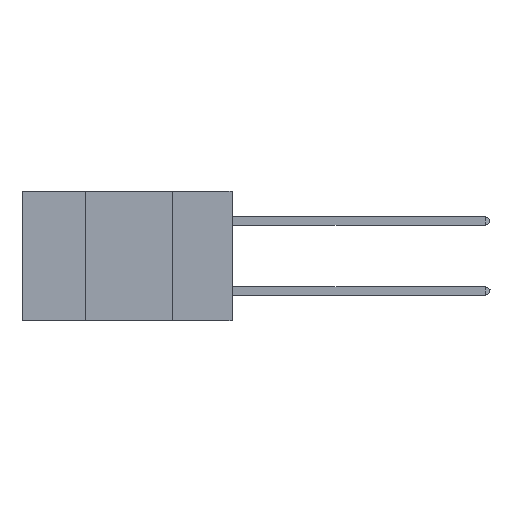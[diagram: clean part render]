
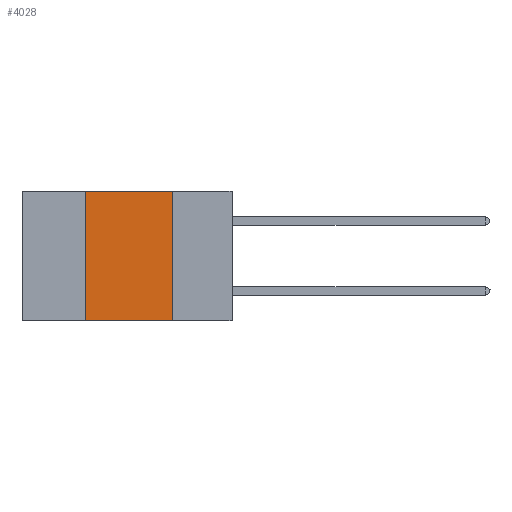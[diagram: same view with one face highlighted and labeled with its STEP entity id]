
A CAD part, left-side view. The second image highlights one B-rep face of the part: STEP entity #4028.
In plain terms, the highlighted planar face has unit normal (-1, 0, 0).
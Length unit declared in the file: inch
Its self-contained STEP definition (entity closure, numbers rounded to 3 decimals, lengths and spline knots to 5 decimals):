
#458 = DIRECTION ( 'NONE',  ( 0., -1., 0. ) ) ;
#980 = CARTESIAN_POINT ( 'NONE',  ( 0., 0.17, 0. ) ) ;
#1110 = DIRECTION ( 'NONE',  ( 0., 0., -1. ) ) ;
#1674 = AXIS2_PLACEMENT_3D ( 'NONE', #3678, #12924, #1110 ) ;
#2007 = ORIENTED_EDGE ( 'NONE', *, *, #4683, .F. ) ;
#3109 = CARTESIAN_POINT ( 'NONE',  ( 0., 0.6, -0.37 ) ) ;
#3633 = CARTESIAN_POINT ( 'NONE',  ( 0., 0.6, 0. ) ) ;
#3663 = VERTEX_POINT ( 'NONE', #13296 ) ;
#3672 = DIRECTION ( 'NONE',  ( 0., 0., -1. ) ) ;
#3678 = CARTESIAN_POINT ( 'NONE',  ( 0., 0.6, 0. ) ) ;
#3947 = DIRECTION ( 'NONE',  ( 0., 0., 1. ) ) ;
#4014 = DIRECTION ( 'NONE',  ( 0., -1., 0. ) ) ;
#4028 = ADVANCED_FACE ( 'NONE', ( #15529 ), #5142, .F. ) ;
#4683 = EDGE_CURVE ( 'NONE', #16263, #7193, #15882, .T. ) ;
#4981 = LINE ( 'NONE', #3633, #12598 ) ;
#5142 = PLANE ( 'NONE',  #1674 ) ;
#5556 = CARTESIAN_POINT ( 'NONE',  ( 0., 0.17, 0. ) ) ;
#5921 = CARTESIAN_POINT ( 'NONE',  ( 0., 0.17, -0.37 ) ) ;
#6955 = VECTOR ( 'NONE', #3672, 39.37008 ) ;
#7193 = VERTEX_POINT ( 'NONE', #5921 ) ;
#7701 = CARTESIAN_POINT ( 'NONE',  ( 0., 0.42, 0. ) ) ;
#8102 = EDGE_CURVE ( 'NONE', #11005, #7193, #16349, .T. ) ;
#8634 = VECTOR ( 'NONE', #458, 39.37008 ) ;
#11005 = VERTEX_POINT ( 'NONE', #14787 ) ;
#12093 = VECTOR ( 'NONE', #3947, 39.37008 ) ;
#12598 = VECTOR ( 'NONE', #4014, 39.37008 ) ;
#12666 = ORIENTED_EDGE ( 'NONE', *, *, #8102, .T. ) ;
#12924 = DIRECTION ( 'NONE',  ( 1., 0., 0. ) ) ;
#13296 = CARTESIAN_POINT ( 'NONE',  ( 0., 0.42, 0. ) ) ;
#14787 = CARTESIAN_POINT ( 'NONE',  ( 0., 0.42, -0.37 ) ) ;
#15362 = EDGE_CURVE ( 'NONE', #3663, #16263, #4981, .T. ) ;
#15529 = FACE_OUTER_BOUND ( 'NONE', #15834, .T. ) ;
#15834 = EDGE_LOOP ( 'NONE', ( #2007, #16234, #16382, #12666 ) ) ;
#15882 = LINE ( 'NONE', #980, #6955 ) ;
#16234 = ORIENTED_EDGE ( 'NONE', *, *, #15362, .F. ) ;
#16263 = VERTEX_POINT ( 'NONE', #5556 ) ;
#16349 = LINE ( 'NONE', #3109, #8634 ) ;
#16382 = ORIENTED_EDGE ( 'NONE', *, *, #17035, .F. ) ;
#16722 = LINE ( 'NONE', #7701, #12093 ) ;
#17035 = EDGE_CURVE ( 'NONE', #11005, #3663, #16722, .T. ) ;
